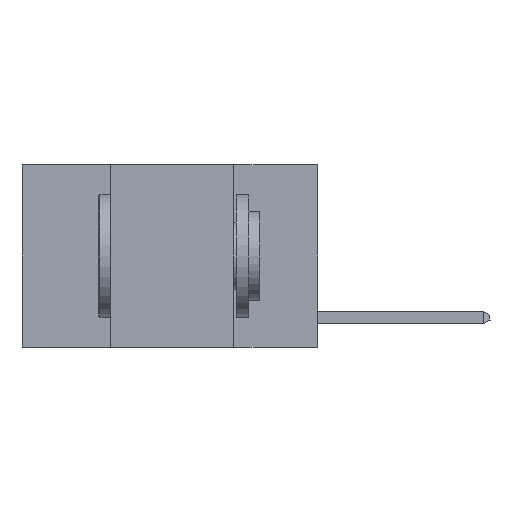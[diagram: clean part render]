
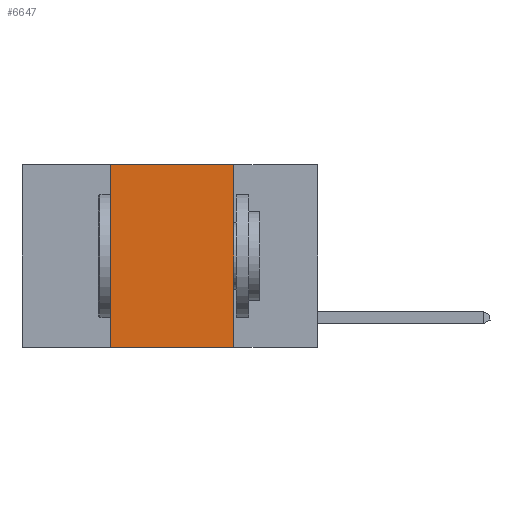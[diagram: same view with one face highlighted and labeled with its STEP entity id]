
A CAD part, left-side view. The second image highlights one B-rep face of the part: STEP entity #6647.
In plain terms, the highlighted planar face has unit normal (-1, 0, 0).
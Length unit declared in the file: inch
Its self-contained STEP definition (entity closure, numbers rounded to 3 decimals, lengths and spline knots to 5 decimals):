
#122 = CARTESIAN_POINT ( 'NONE',  ( 0., 0.17, -0.37 ) ) ;
#514 = LINE ( 'NONE', #1653, #9187 ) ;
#1653 = CARTESIAN_POINT ( 'NONE',  ( 0., 0.42, 0. ) ) ;
#1879 = DIRECTION ( 'NONE',  ( 0., -1., 0. ) ) ;
#2023 = VERTEX_POINT ( 'NONE', #17518 ) ;
#2302 = CARTESIAN_POINT ( 'NONE',  ( 0., 0.17, 0. ) ) ;
#3424 = DIRECTION ( 'NONE',  ( 0., 0., 1. ) ) ;
#3739 = ORIENTED_EDGE ( 'NONE', *, *, #8506, .F. ) ;
#4087 = VECTOR ( 'NONE', #5746, 39.37008 ) ;
#5582 = PLANE ( 'NONE',  #8452 ) ;
#5746 = DIRECTION ( 'NONE',  ( 0., 0., -1. ) ) ;
#5788 = DIRECTION ( 'NONE',  ( 0., -1., 0. ) ) ;
#5824 = VERTEX_POINT ( 'NONE', #19580 ) ;
#6647 = ADVANCED_FACE ( 'NONE', ( #11359 ), #5582, .F. ) ;
#7340 = DIRECTION ( 'NONE',  ( 1., 0., 0. ) ) ;
#7406 = EDGE_CURVE ( 'NONE', #5824, #17733, #18418, .T. ) ;
#7599 = VECTOR ( 'NONE', #1879, 39.37008 ) ;
#8302 = ORIENTED_EDGE ( 'NONE', *, *, #7406, .F. ) ;
#8452 = AXIS2_PLACEMENT_3D ( 'NONE', #15722, #7340, #19068 ) ;
#8506 = EDGE_CURVE ( 'NONE', #17733, #16382, #13114, .T. ) ;
#8842 = ORIENTED_EDGE ( 'NONE', *, *, #15004, .F. ) ;
#9187 = VECTOR ( 'NONE', #3424, 39.37008 ) ;
#10825 = CARTESIAN_POINT ( 'NONE',  ( 0., 0.6, 0. ) ) ;
#11359 = FACE_OUTER_BOUND ( 'NONE', #19818, .T. ) ;
#13114 = LINE ( 'NONE', #17457, #4087 ) ;
#15004 = EDGE_CURVE ( 'NONE', #2023, #5824, #514, .T. ) ;
#15106 = EDGE_CURVE ( 'NONE', #2023, #16382, #20971, .T. ) ;
#15722 = CARTESIAN_POINT ( 'NONE',  ( 0., 0.6, 0. ) ) ;
#16382 = VERTEX_POINT ( 'NONE', #122 ) ;
#17457 = CARTESIAN_POINT ( 'NONE',  ( 0., 0.17, 0. ) ) ;
#17518 = CARTESIAN_POINT ( 'NONE',  ( 0., 0.42, -0.37 ) ) ;
#17733 = VERTEX_POINT ( 'NONE', #2302 ) ;
#17760 = ORIENTED_EDGE ( 'NONE', *, *, #15106, .T. ) ;
#17887 = VECTOR ( 'NONE', #5788, 39.37008 ) ;
#18418 = LINE ( 'NONE', #10825, #17887 ) ;
#19068 = DIRECTION ( 'NONE',  ( 0., 0., -1. ) ) ;
#19580 = CARTESIAN_POINT ( 'NONE',  ( 0., 0.42, 0. ) ) ;
#19818 = EDGE_LOOP ( 'NONE', ( #3739, #8302, #8842, #17760 ) ) ;
#20474 = CARTESIAN_POINT ( 'NONE',  ( 0., 0.6, -0.37 ) ) ;
#20971 = LINE ( 'NONE', #20474, #7599 ) ;
